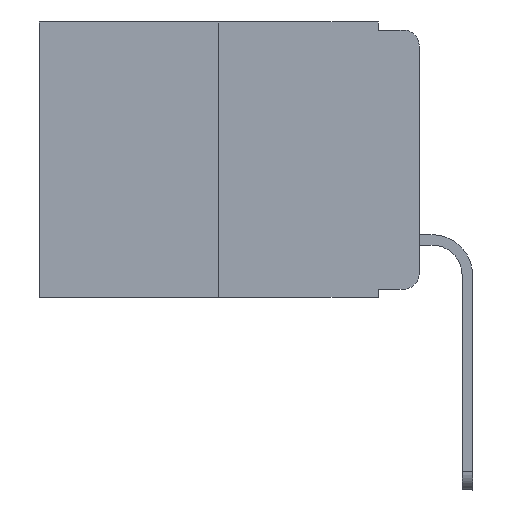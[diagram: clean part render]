
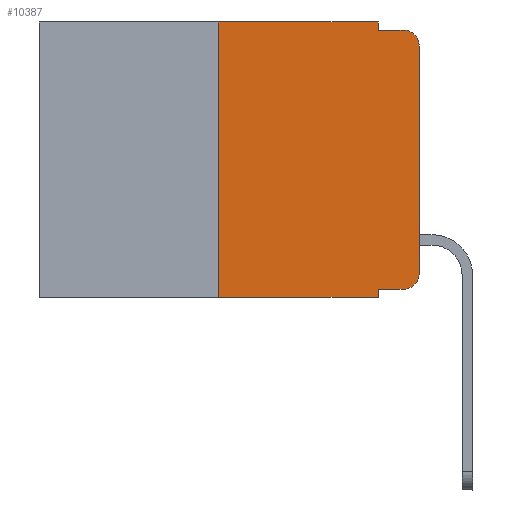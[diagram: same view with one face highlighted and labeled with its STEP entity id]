
A CAD part, left-side view. The second image highlights one B-rep face of the part: STEP entity #10387.
In plain terms, the highlighted planar face has unit normal (-1, 0, 0).
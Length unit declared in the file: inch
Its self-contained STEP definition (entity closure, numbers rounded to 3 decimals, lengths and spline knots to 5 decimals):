
#37 = CARTESIAN_POINT ( 'NONE',  ( 0., 0.051, -0.01 ) ) ;
#139 = VERTEX_POINT ( 'NONE', #12741 ) ;
#261 = EDGE_CURVE ( 'NONE', #5722, #4982, #13012, .T. ) ;
#361 = VERTEX_POINT ( 'NONE', #5517 ) ;
#388 = ORIENTED_EDGE ( 'NONE', *, *, #10171, .F. ) ;
#405 = LINE ( 'NONE', #13577, #9818 ) ;
#411 = AXIS2_PLACEMENT_3D ( 'NONE', #1642, #1508, #6980 ) ;
#420 = CARTESIAN_POINT ( 'NONE',  ( 0., 0.051, 0. ) ) ;
#618 = DIRECTION ( 'NONE',  ( 0., 0., -1. ) ) ;
#1127 = DIRECTION ( 'NONE',  ( 0., -1., 0. ) ) ;
#1237 = LINE ( 'NONE', #2225, #11377 ) ;
#1339 = DIRECTION ( 'NONE',  ( 0., 0., -1. ) ) ;
#1413 = ORIENTED_EDGE ( 'NONE', *, *, #5080, .T. ) ;
#1508 = DIRECTION ( 'NONE',  ( -1., 0., 0. ) ) ;
#1642 = CARTESIAN_POINT ( 'NONE',  ( 0., 0.02, -0.03 ) ) ;
#1697 = VECTOR ( 'NONE', #1127, 39.37008 ) ;
#1972 = DIRECTION ( 'NONE',  ( 0., 0., -1. ) ) ;
#2069 = ORIENTED_EDGE ( 'NONE', *, *, #4231, .T. ) ;
#2144 = VERTEX_POINT ( 'NONE', #10928 ) ;
#2225 = CARTESIAN_POINT ( 'NONE',  ( 0., 0.051, -0.333 ) ) ;
#2378 = EDGE_LOOP ( 'NONE', ( #2772, #2069, #4194, #388, #9443, #12819, #1413, #5059, #5467, #4819 ) ) ;
#2539 = CARTESIAN_POINT ( 'NONE',  ( 0., 0.051, 0. ) ) ;
#2622 = CARTESIAN_POINT ( 'NONE',  ( 0., 0.02, -0.313 ) ) ;
#2772 = ORIENTED_EDGE ( 'NONE', *, *, #5965, .T. ) ;
#2964 = CARTESIAN_POINT ( 'NONE',  ( 0., 0., 0. ) ) ;
#2993 = EDGE_CURVE ( 'NONE', #8018, #2144, #13030, .T. ) ;
#3535 = DIRECTION ( 'NONE',  ( 0., -1., 0. ) ) ;
#3637 = VECTOR ( 'NONE', #618, 39.37008 ) ;
#3898 = AXIS2_PLACEMENT_3D ( 'NONE', #6431, #11747, #1972 ) ;
#4053 = AXIS2_PLACEMENT_3D ( 'NONE', #2622, #7947, #7037 ) ;
#4110 = LINE ( 'NONE', #2964, #9262 ) ;
#4194 = ORIENTED_EDGE ( 'NONE', *, *, #2993, .F. ) ;
#4231 = EDGE_CURVE ( 'NONE', #361, #2144, #10201, .T. ) ;
#4243 = CARTESIAN_POINT ( 'NONE',  ( 0., 0.25, 0. ) ) ;
#4546 = EDGE_CURVE ( 'NONE', #13420, #6076, #5879, .T. ) ;
#4754 = LINE ( 'NONE', #2539, #3637 ) ;
#4819 = ORIENTED_EDGE ( 'NONE', *, *, #4546, .T. ) ;
#4982 = VERTEX_POINT ( 'NONE', #5819 ) ;
#5059 = ORIENTED_EDGE ( 'NONE', *, *, #7567, .F. ) ;
#5069 = CARTESIAN_POINT ( 'NONE',  ( 0., 0.051, -0.343 ) ) ;
#5080 = EDGE_CURVE ( 'NONE', #5722, #5524, #405, .T. ) ;
#5235 = CARTESIAN_POINT ( 'NONE',  ( 0., 0.051, -0.01 ) ) ;
#5236 = VERTEX_POINT ( 'NONE', #8622 ) ;
#5467 = ORIENTED_EDGE ( 'NONE', *, *, #7827, .T. ) ;
#5517 = CARTESIAN_POINT ( 'NONE',  ( 0., 0., -0.03 ) ) ;
#5524 = VERTEX_POINT ( 'NONE', #5069 ) ;
#5722 = VERTEX_POINT ( 'NONE', #13318 ) ;
#5819 = CARTESIAN_POINT ( 'NONE',  ( 0., 0.25, 0. ) ) ;
#5879 = CIRCLE ( 'NONE', #4053, 0.02 ) ;
#5965 = EDGE_CURVE ( 'NONE', #6076, #361, #4110, .T. ) ;
#6076 = VERTEX_POINT ( 'NONE', #8526 ) ;
#6431 = CARTESIAN_POINT ( 'NONE',  ( 0., 0.473, 0. ) ) ;
#6823 = LINE ( 'NONE', #420, #11195 ) ;
#6846 = LINE ( 'NONE', #7189, #11853 ) ;
#6980 = DIRECTION ( 'NONE',  ( 0., 0., -1. ) ) ;
#7037 = DIRECTION ( 'NONE',  ( 0., 0., -1. ) ) ;
#7089 = EDGE_CURVE ( 'NONE', #4982, #139, #6846, .T. ) ;
#7189 = CARTESIAN_POINT ( 'NONE',  ( 0., 0.473, 0. ) ) ;
#7567 = EDGE_CURVE ( 'NONE', #5236, #5524, #4754, .T. ) ;
#7827 = EDGE_CURVE ( 'NONE', #5236, #13420, #1237, .T. ) ;
#7947 = DIRECTION ( 'NONE',  ( -1., 0., 0. ) ) ;
#8018 = VERTEX_POINT ( 'NONE', #5235 ) ;
#8359 = PLANE ( 'NONE',  #3898 ) ;
#8526 = CARTESIAN_POINT ( 'NONE',  ( 0., 0., -0.313 ) ) ;
#8622 = CARTESIAN_POINT ( 'NONE',  ( 0., 0.051, -0.333 ) ) ;
#9262 = VECTOR ( 'NONE', #13950, 39.37008 ) ;
#9443 = ORIENTED_EDGE ( 'NONE', *, *, #7089, .F. ) ;
#9818 = VECTOR ( 'NONE', #3535, 39.37008 ) ;
#10171 = EDGE_CURVE ( 'NONE', #139, #8018, #6823, .T. ) ;
#10201 = CIRCLE ( 'NONE', #411, 0.02 ) ;
#10387 = ADVANCED_FACE ( 'NONE', ( #12671 ), #8359, .F. ) ;
#10928 = CARTESIAN_POINT ( 'NONE',  ( 0., 0.02, -0.01 ) ) ;
#11195 = VECTOR ( 'NONE', #1339, 39.37008 ) ;
#11224 = VECTOR ( 'NONE', #12939, 39.37008 ) ;
#11230 = DIRECTION ( 'NONE',  ( 0., -1., 0. ) ) ;
#11377 = VECTOR ( 'NONE', #11230, 39.37008 ) ;
#11476 = DIRECTION ( 'NONE',  ( 0., -1., 0. ) ) ;
#11714 = CARTESIAN_POINT ( 'NONE',  ( 0., 0.02, -0.333 ) ) ;
#11747 = DIRECTION ( 'NONE',  ( 1., 0., 0. ) ) ;
#11853 = VECTOR ( 'NONE', #11476, 39.37008 ) ;
#12671 = FACE_OUTER_BOUND ( 'NONE', #2378, .T. ) ;
#12741 = CARTESIAN_POINT ( 'NONE',  ( 0., 0.051, 0. ) ) ;
#12819 = ORIENTED_EDGE ( 'NONE', *, *, #261, .F. ) ;
#12939 = DIRECTION ( 'NONE',  ( 0., 0., 1. ) ) ;
#13012 = LINE ( 'NONE', #4243, #11224 ) ;
#13030 = LINE ( 'NONE', #37, #1697 ) ;
#13318 = CARTESIAN_POINT ( 'NONE',  ( 0., 0.25, -0.343 ) ) ;
#13420 = VERTEX_POINT ( 'NONE', #11714 ) ;
#13577 = CARTESIAN_POINT ( 'NONE',  ( 0., 0.473, -0.343 ) ) ;
#13950 = DIRECTION ( 'NONE',  ( 0., 0., 1. ) ) ;
